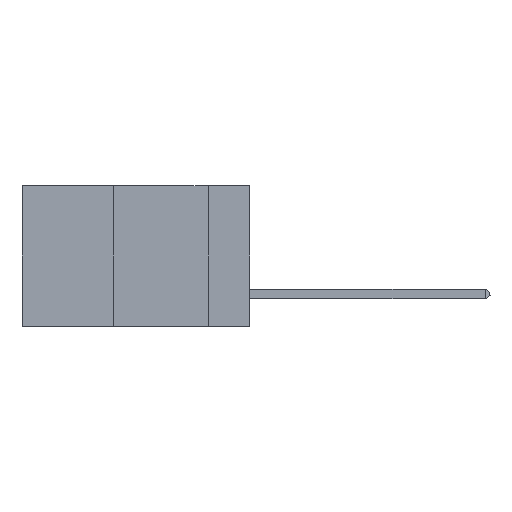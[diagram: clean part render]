
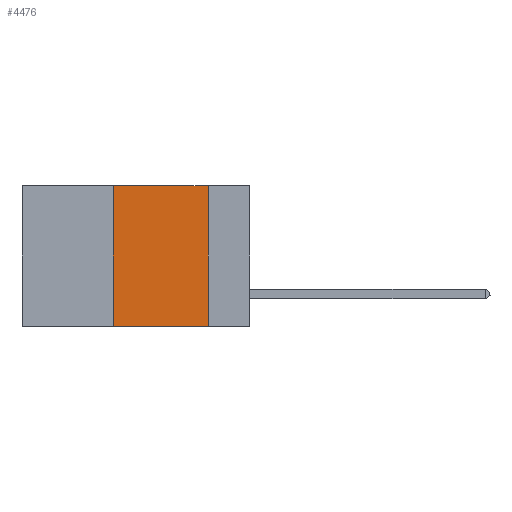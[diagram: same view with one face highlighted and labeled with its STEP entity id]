
A CAD part, left-side view. The second image highlights one B-rep face of the part: STEP entity #4476.
In plain terms, the highlighted planar face has unit normal (-1, 0, 0).
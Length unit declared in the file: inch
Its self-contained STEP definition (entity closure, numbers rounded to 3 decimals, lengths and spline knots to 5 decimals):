
#1151 = CARTESIAN_POINT ( 'NONE',  ( 0., 0.11, -0.37 ) ) ;
#1617 = EDGE_CURVE ( 'NONE', #22767, #13380, #19523, .T. ) ;
#4476 = ADVANCED_FACE ( 'NONE', ( #25738 ), #20995, .F. ) ;
#4773 = DIRECTION ( 'NONE',  ( 0., -1., 0. ) ) ;
#7268 = VECTOR ( 'NONE', #14094, 39.37008 ) ;
#7460 = CARTESIAN_POINT ( 'NONE',  ( 0., 0.36, 0. ) ) ;
#8817 = CARTESIAN_POINT ( 'NONE',  ( 0., 0.36, 0. ) ) ;
#9590 = CARTESIAN_POINT ( 'NONE',  ( 0., 0.6, 0. ) ) ;
#9750 = VECTOR ( 'NONE', #18430, 39.37008 ) ;
#10560 = EDGE_CURVE ( 'NONE', #18055, #22767, #24565, .T. ) ;
#10781 = ORIENTED_EDGE ( 'NONE', *, *, #21213, .F. ) ;
#13380 = VERTEX_POINT ( 'NONE', #1151 ) ;
#13405 = DIRECTION ( 'NONE',  ( 1., 0., 0. ) ) ;
#13583 = CARTESIAN_POINT ( 'NONE',  ( 0., 0.6, -0.37 ) ) ;
#13687 = ORIENTED_EDGE ( 'NONE', *, *, #10560, .F. ) ;
#14094 = DIRECTION ( 'NONE',  ( 0., 0., 1. ) ) ;
#17109 = CARTESIAN_POINT ( 'NONE',  ( 0., 0.36, -0.37 ) ) ;
#17145 = EDGE_CURVE ( 'NONE', #23202, #13380, #21944, .T. ) ;
#18055 = VERTEX_POINT ( 'NONE', #7460 ) ;
#18212 = CARTESIAN_POINT ( 'NONE',  ( 0., 0.11, 0. ) ) ;
#18357 = DIRECTION ( 'NONE',  ( 0., 0., -1. ) ) ;
#18430 = DIRECTION ( 'NONE',  ( 0., 0., -1. ) ) ;
#19312 = ORIENTED_EDGE ( 'NONE', *, *, #1617, .F. ) ;
#19339 = VECTOR ( 'NONE', #4773, 39.37008 ) ;
#19364 = VECTOR ( 'NONE', #26269, 39.37008 ) ;
#19523 = LINE ( 'NONE', #18212, #9750 ) ;
#19626 = LINE ( 'NONE', #8817, #7268 ) ;
#20995 = PLANE ( 'NONE',  #28010 ) ;
#21213 = EDGE_CURVE ( 'NONE', #23202, #18055, #19626, .T. ) ;
#21944 = LINE ( 'NONE', #13583, #19364 ) ;
#22767 = VERTEX_POINT ( 'NONE', #27322 ) ;
#23202 = VERTEX_POINT ( 'NONE', #17109 ) ;
#23216 = CARTESIAN_POINT ( 'NONE',  ( 0., 0.6, 0. ) ) ;
#24565 = LINE ( 'NONE', #9590, #19339 ) ;
#24856 = EDGE_LOOP ( 'NONE', ( #19312, #13687, #10781, #29841 ) ) ;
#25738 = FACE_OUTER_BOUND ( 'NONE', #24856, .T. ) ;
#26269 = DIRECTION ( 'NONE',  ( 0., -1., 0. ) ) ;
#27322 = CARTESIAN_POINT ( 'NONE',  ( 0., 0.11, 0. ) ) ;
#28010 = AXIS2_PLACEMENT_3D ( 'NONE', #23216, #13405, #18357 ) ;
#29841 = ORIENTED_EDGE ( 'NONE', *, *, #17145, .T. ) ;
